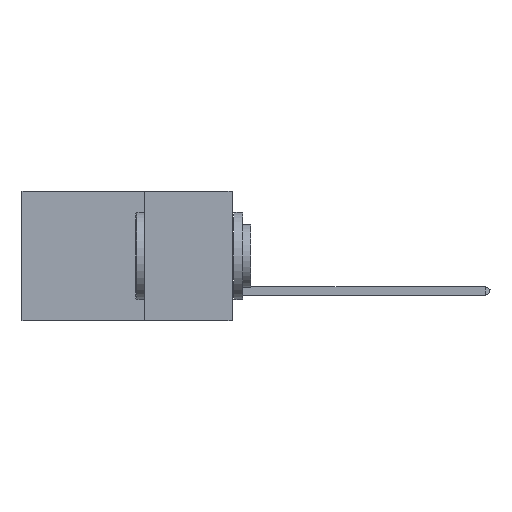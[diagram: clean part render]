
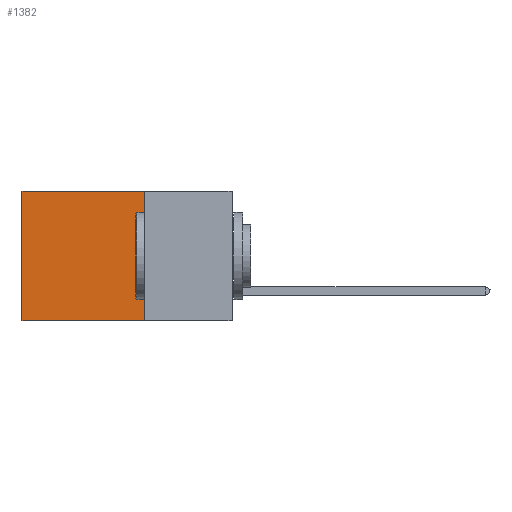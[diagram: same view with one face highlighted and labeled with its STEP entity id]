
A CAD part, left-side view. The second image highlights one B-rep face of the part: STEP entity #1382.
In plain terms, the highlighted planar face has unit normal (-1, 0, 0).
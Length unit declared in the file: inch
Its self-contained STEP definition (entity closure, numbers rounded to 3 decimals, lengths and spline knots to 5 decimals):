
#1061 = CARTESIAN_POINT ( 'NONE',  ( 0.2875, 0.25, -0.37 ) ) ;
#1066 = CARTESIAN_POINT ( 'NONE',  ( 0.2875, 0.25, -0.37 ) ) ;
#1382 = ADVANCED_FACE ( 'NONE', ( #13914 ), #19484, .F. ) ;
#3617 = VECTOR ( 'NONE', #3929, 39.37008 ) ;
#3929 = DIRECTION ( 'NONE',  ( 0., 0., -1. ) ) ;
#4265 = EDGE_CURVE ( 'NONE', #6158, #14458, #16627, .T. ) ;
#4323 = CARTESIAN_POINT ( 'NONE',  ( 0.2875, 0.25, 0. ) ) ;
#4435 = VERTEX_POINT ( 'NONE', #14622 ) ;
#5409 = EDGE_CURVE ( 'NONE', #14458, #4435, #15851, .T. ) ;
#5857 = DIRECTION ( 'NONE',  ( 1., 0., 0. ) ) ;
#6142 = ORIENTED_EDGE ( 'NONE', *, *, #8266, .F. ) ;
#6158 = VERTEX_POINT ( 'NONE', #18104 ) ;
#7608 = ORIENTED_EDGE ( 'NONE', *, *, #5409, .T. ) ;
#8266 = EDGE_CURVE ( 'NONE', #9256, #4435, #15509, .T. ) ;
#8436 = ORIENTED_EDGE ( 'NONE', *, *, #11727, .F. ) ;
#8645 = VECTOR ( 'NONE', #14939, 39.37008 ) ;
#8980 = DIRECTION ( 'NONE',  ( 0., 0., -1. ) ) ;
#9256 = VERTEX_POINT ( 'NONE', #1066 ) ;
#11727 = EDGE_CURVE ( 'NONE', #6158, #9256, #11754, .T. ) ;
#11754 = LINE ( 'NONE', #14530, #3617 ) ;
#12441 = EDGE_LOOP ( 'NONE', ( #7608, #6142, #8436, #12761 ) ) ;
#12761 = ORIENTED_EDGE ( 'NONE', *, *, #4265, .T. ) ;
#13914 = FACE_OUTER_BOUND ( 'NONE', #12441, .T. ) ;
#13926 = CARTESIAN_POINT ( 'NONE',  ( 0.2875, 0.25, 0. ) ) ;
#14083 = CARTESIAN_POINT ( 'NONE',  ( 0.2875, 0.6, 0. ) ) ;
#14458 = VERTEX_POINT ( 'NONE', #14083 ) ;
#14530 = CARTESIAN_POINT ( 'NONE',  ( 0.2875, 0.25, 0. ) ) ;
#14622 = CARTESIAN_POINT ( 'NONE',  ( 0.2875, 0.6, -0.37 ) ) ;
#14724 = VECTOR ( 'NONE', #18426, 39.37008 ) ;
#14939 = DIRECTION ( 'NONE',  ( 0., 1., 0. ) ) ;
#15509 = LINE ( 'NONE', #1061, #8645 ) ;
#15851 = LINE ( 'NONE', #16006, #17287 ) ;
#16006 = CARTESIAN_POINT ( 'NONE',  ( 0.2875, 0.6, 0. ) ) ;
#16502 = AXIS2_PLACEMENT_3D ( 'NONE', #4323, #5857, #8980 ) ;
#16627 = LINE ( 'NONE', #13926, #14724 ) ;
#17287 = VECTOR ( 'NONE', #19125, 39.37008 ) ;
#18104 = CARTESIAN_POINT ( 'NONE',  ( 0.2875, 0.25, 0. ) ) ;
#18426 = DIRECTION ( 'NONE',  ( 0., 1., 0. ) ) ;
#19125 = DIRECTION ( 'NONE',  ( 0., 0., -1. ) ) ;
#19484 = PLANE ( 'NONE',  #16502 ) ;
